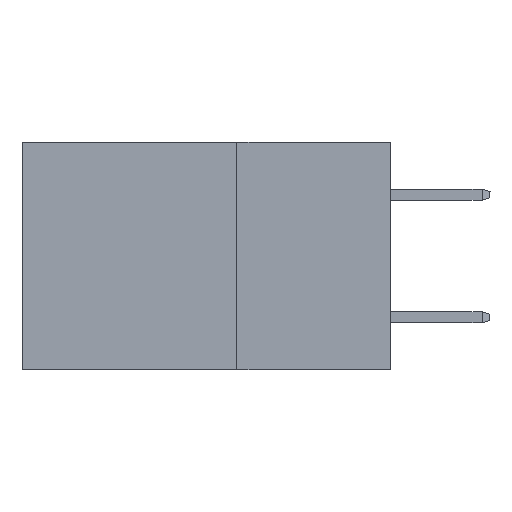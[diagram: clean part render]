
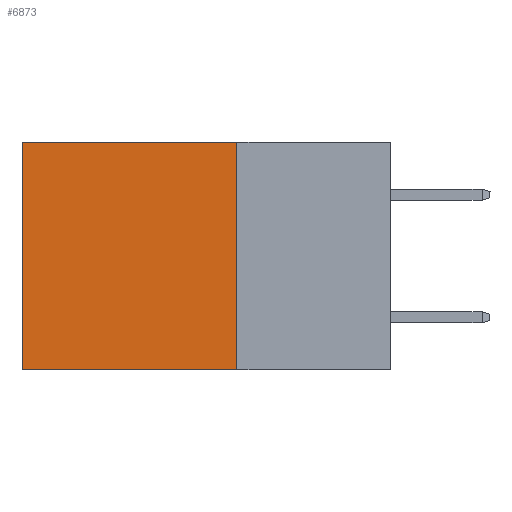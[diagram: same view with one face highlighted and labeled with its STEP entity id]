
A CAD part, left-side view. The second image highlights one B-rep face of the part: STEP entity #6873.
In plain terms, the highlighted planar face has unit normal (-1, 0, 0).
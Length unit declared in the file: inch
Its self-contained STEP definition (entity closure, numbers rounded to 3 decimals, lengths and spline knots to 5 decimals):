
#293 = LINE ( 'NONE', #5605, #6821 ) ;
#663 = VECTOR ( 'NONE', #6726, 39.37008 ) ;
#673 = ORIENTED_EDGE ( 'NONE', *, *, #4602, .T. ) ;
#759 = PLANE ( 'NONE',  #4620 ) ;
#769 = CARTESIAN_POINT ( 'NONE',  ( 0.2875, 0.25, 0. ) ) ;
#1231 = DIRECTION ( 'NONE',  ( 0., 1., 0. ) ) ;
#1322 = VECTOR ( 'NONE', #8541, 39.37008 ) ;
#1758 = LINE ( 'NONE', #8685, #663 ) ;
#2291 = EDGE_CURVE ( 'NONE', #4751, #4778, #12027, .T. ) ;
#2360 = CARTESIAN_POINT ( 'NONE',  ( 0.2875, 0.25, -0.37 ) ) ;
#3168 = CARTESIAN_POINT ( 'NONE',  ( 0.2875, 0.25, -0.37 ) ) ;
#3638 = DIRECTION ( 'NONE',  ( 0., 0., -1. ) ) ;
#3763 = DIRECTION ( 'NONE',  ( 1., 0., 0. ) ) ;
#4602 = EDGE_CURVE ( 'NONE', #4619, #4778, #293, .T. ) ;
#4619 = VERTEX_POINT ( 'NONE', #4720 ) ;
#4620 = AXIS2_PLACEMENT_3D ( 'NONE', #9728, #3763, #3638 ) ;
#4720 = CARTESIAN_POINT ( 'NONE',  ( 0.2875, 0.6, 0. ) ) ;
#4751 = VERTEX_POINT ( 'NONE', #3168 ) ;
#4778 = VERTEX_POINT ( 'NONE', #5284 ) ;
#5284 = CARTESIAN_POINT ( 'NONE',  ( 0.2875, 0.6, -0.37 ) ) ;
#5605 = CARTESIAN_POINT ( 'NONE',  ( 0.2875, 0.6, 0. ) ) ;
#6726 = DIRECTION ( 'NONE',  ( 0., 0., -1. ) ) ;
#6796 = EDGE_CURVE ( 'NONE', #10130, #4619, #6919, .T. ) ;
#6821 = VECTOR ( 'NONE', #10610, 39.37008 ) ;
#6873 = ADVANCED_FACE ( 'NONE', ( #12387 ), #759, .F. ) ;
#6919 = LINE ( 'NONE', #12519, #1322 ) ;
#7980 = EDGE_LOOP ( 'NONE', ( #673, #10005, #11502, #8391 ) ) ;
#8161 = EDGE_CURVE ( 'NONE', #10130, #4751, #1758, .T. ) ;
#8391 = ORIENTED_EDGE ( 'NONE', *, *, #6796, .T. ) ;
#8541 = DIRECTION ( 'NONE',  ( 0., 1., 0. ) ) ;
#8685 = CARTESIAN_POINT ( 'NONE',  ( 0.2875, 0.25, 0. ) ) ;
#9728 = CARTESIAN_POINT ( 'NONE',  ( 0.2875, 0.25, 0. ) ) ;
#10005 = ORIENTED_EDGE ( 'NONE', *, *, #2291, .F. ) ;
#10130 = VERTEX_POINT ( 'NONE', #769 ) ;
#10610 = DIRECTION ( 'NONE',  ( 0., 0., -1. ) ) ;
#11502 = ORIENTED_EDGE ( 'NONE', *, *, #8161, .F. ) ;
#12027 = LINE ( 'NONE', #2360, #12809 ) ;
#12387 = FACE_OUTER_BOUND ( 'NONE', #7980, .T. ) ;
#12519 = CARTESIAN_POINT ( 'NONE',  ( 0.2875, 0.25, 0. ) ) ;
#12809 = VECTOR ( 'NONE', #1231, 39.37008 ) ;
